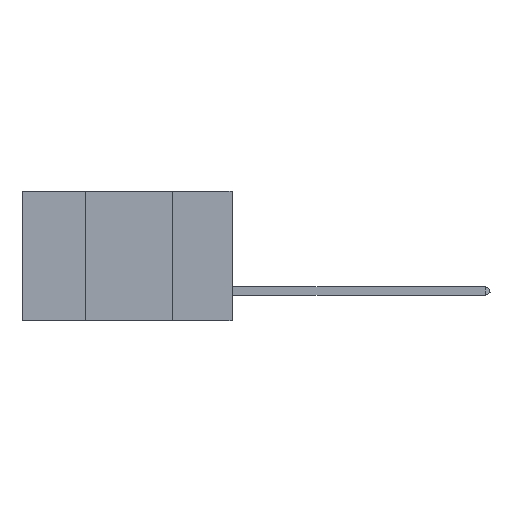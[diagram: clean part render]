
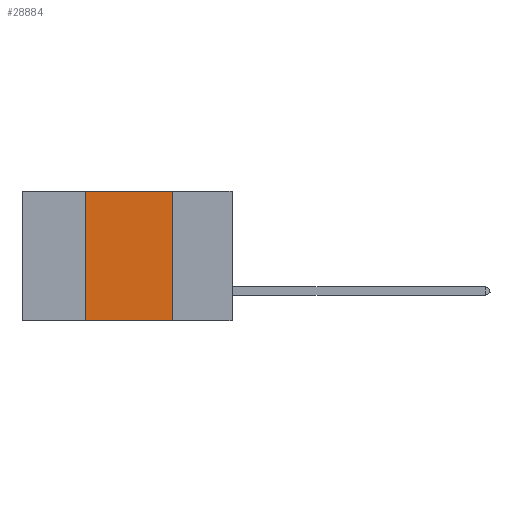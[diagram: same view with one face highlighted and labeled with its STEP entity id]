
A CAD part, left-side view. The second image highlights one B-rep face of the part: STEP entity #28884.
In plain terms, the highlighted planar face has unit normal (-1, 0, 0).
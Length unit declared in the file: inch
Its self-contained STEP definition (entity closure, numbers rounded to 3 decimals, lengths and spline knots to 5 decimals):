
#1312 = EDGE_CURVE ( 'NONE', #33284, #2899, #15805, .T. ) ;
#1970 = VECTOR ( 'NONE', #18227, 39.37008 ) ;
#2168 = LINE ( 'NONE', #15326, #9112 ) ;
#2899 = VERTEX_POINT ( 'NONE', #18553 ) ;
#2976 = EDGE_LOOP ( 'NONE', ( #10027, #21983, #3749, #16748 ) ) ;
#3521 = VECTOR ( 'NONE', #26041, 39.37008 ) ;
#3749 = ORIENTED_EDGE ( 'NONE', *, *, #13029, .F. ) ;
#3923 = AXIS2_PLACEMENT_3D ( 'NONE', #14549, #12259, #11924 ) ;
#5155 = CARTESIAN_POINT ( 'NONE',  ( 0., 0.17, -0.37 ) ) ;
#6287 = FACE_OUTER_BOUND ( 'NONE', #2976, .T. ) ;
#8860 = VERTEX_POINT ( 'NONE', #13639 ) ;
#9112 = VECTOR ( 'NONE', #25405, 39.37008 ) ;
#9229 = CARTESIAN_POINT ( 'NONE',  ( 0., 0.42, 0. ) ) ;
#9550 = EDGE_CURVE ( 'NONE', #8860, #23818, #25606, .T. ) ;
#10027 = ORIENTED_EDGE ( 'NONE', *, *, #24402, .F. ) ;
#10719 = DIRECTION ( 'NONE',  ( 0., -1., 0. ) ) ;
#11033 = VECTOR ( 'NONE', #10719, 39.37008 ) ;
#11924 = DIRECTION ( 'NONE',  ( 0., 0., -1. ) ) ;
#12259 = DIRECTION ( 'NONE',  ( 1., 0., 0. ) ) ;
#13029 = EDGE_CURVE ( 'NONE', #8860, #33284, #31106, .T. ) ;
#13639 = CARTESIAN_POINT ( 'NONE',  ( 0., 0.42, -0.37 ) ) ;
#14549 = CARTESIAN_POINT ( 'NONE',  ( 0., 0.6, 0. ) ) ;
#15326 = CARTESIAN_POINT ( 'NONE',  ( 0., 0.17, 0. ) ) ;
#15805 = LINE ( 'NONE', #20351, #1970 ) ;
#16748 = ORIENTED_EDGE ( 'NONE', *, *, #9550, .T. ) ;
#18227 = DIRECTION ( 'NONE',  ( 0., -1., 0. ) ) ;
#18553 = CARTESIAN_POINT ( 'NONE',  ( 0., 0.17, 0. ) ) ;
#20351 = CARTESIAN_POINT ( 'NONE',  ( 0., 0.6, 0. ) ) ;
#21983 = ORIENTED_EDGE ( 'NONE', *, *, #1312, .F. ) ;
#23818 = VERTEX_POINT ( 'NONE', #5155 ) ;
#24402 = EDGE_CURVE ( 'NONE', #2899, #23818, #2168, .T. ) ;
#25405 = DIRECTION ( 'NONE',  ( 0., 0., -1. ) ) ;
#25606 = LINE ( 'NONE', #31020, #11033 ) ;
#26041 = DIRECTION ( 'NONE',  ( 0., 0., 1. ) ) ;
#28884 = ADVANCED_FACE ( 'NONE', ( #6287 ), #30287, .F. ) ;
#30287 = PLANE ( 'NONE',  #3923 ) ;
#31020 = CARTESIAN_POINT ( 'NONE',  ( 0., 0.6, -0.37 ) ) ;
#31106 = LINE ( 'NONE', #33499, #3521 ) ;
#33284 = VERTEX_POINT ( 'NONE', #9229 ) ;
#33499 = CARTESIAN_POINT ( 'NONE',  ( 0., 0.42, 0. ) ) ;
